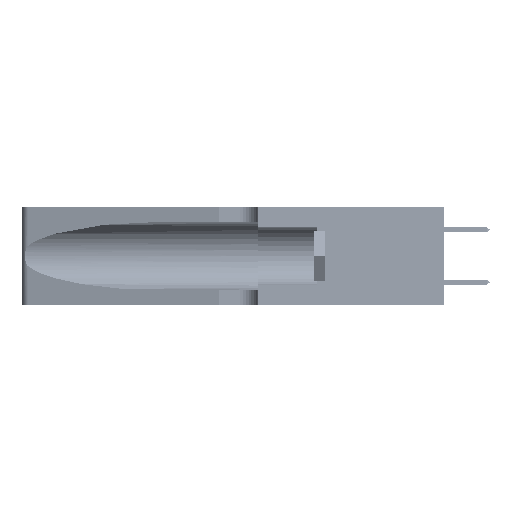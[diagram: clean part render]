
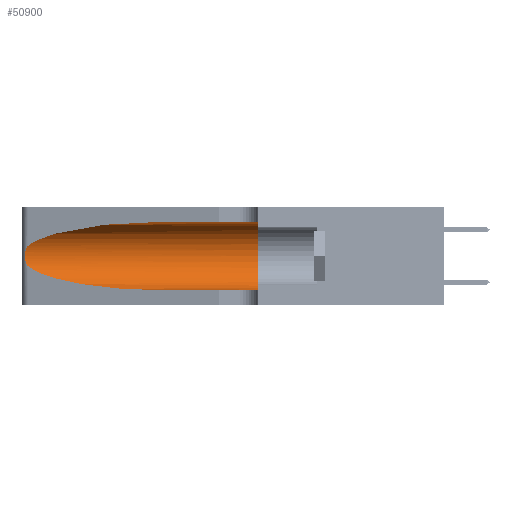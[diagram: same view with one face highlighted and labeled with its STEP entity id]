
A CAD part, left-side view. The second image highlights one B-rep face of the part: STEP entity #50900.
In plain terms, the highlighted cylindrical face has radius 3.308 mm (diameter 6.617 mm), a partial arc.
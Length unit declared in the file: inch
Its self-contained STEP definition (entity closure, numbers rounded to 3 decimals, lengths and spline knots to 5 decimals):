
#383 = CARTESIAN_POINT ( 'NONE',  ( 0.25487, 1.22718, 0.14631 ) ) ;
#480 = DIRECTION ( 'NONE',  ( 0., -1., 0. ) ) ;
#1795 = EDGE_CURVE ( 'NONE', #42013, #22346, #43611, .T. ) ;
#2925 = ORIENTED_EDGE ( 'NONE', *, *, #12198, .T. ) ;
#3217 = CARTESIAN_POINT ( 'NONE',  ( 0.25555, 1.22994, 0.2215 ) ) ;
#3364 = CARTESIAN_POINT ( 'NONE',  ( 0.25487, 1.22718, 0.22369 ) ) ;
#3569 = CARTESIAN_POINT ( 'NONE',  ( 0.25854, 1.2359, 0.20912 ) ) ;
#3576 = VERTEX_POINT ( 'NONE', #20899 ) ;
#4044 = CARTESIAN_POINT ( 'NONE',  ( 0.18966, 0.96281, 0.31525 ) ) ;
#4055 = LINE ( 'NONE', #19057, #10880 ) ;
#4656 = DIRECTION ( 'NONE',  ( 0., 0., -1. ) ) ;
#4986 =( BOUNDED_CURVE ( )  B_SPLINE_CURVE ( 3, ( #47479, #4044, #35626, #3364 ),
 .UNSPECIFIED., .F., .F. ) 
 B_SPLINE_CURVE_WITH_KNOTS ( ( 4, 4 ),
 ( 1.5708, 2.84003 ),
 .UNSPECIFIED. ) 
 CURVE ( )  GEOMETRIC_REPRESENTATION_ITEM ( )  RATIONAL_B_SPLINE_CURVE ( ( 1., 0.87, 0.87, 1. ) ) 
 REPRESENTATION_ITEM ( '' )  );
#7230 = CARTESIAN_POINT ( 'NONE',  ( 0.25487, 1.22718, 0.14631 ) ) ;
#7369 = CARTESIAN_POINT ( 'NONE',  ( 0.26075, 1.23896, 0.178 ) ) ;
#7662 = CYLINDRICAL_SURFACE ( 'NONE', #44489, 0.13025 ) ;
#8273 = CARTESIAN_POINT ( 'NONE',  ( 0.1305, 1.61858, 0.31525 ) ) ;
#9324 = EDGE_CURVE ( 'NONE', #22346, #3576, #16330, .T. ) ;
#10697 = CARTESIAN_POINT ( 'NONE',  ( 0.26017, 1.23833, 0.17102 ) ) ;
#10880 = VECTOR ( 'NONE', #31592, 39.37008 ) ;
#11208 = CARTESIAN_POINT ( 'NONE',  ( 0.25487, 1.22718, 0.14631 ) ) ;
#12198 = EDGE_CURVE ( 'NONE', #37770, #3576, #4055, .T. ) ;
#12504 = DIRECTION ( 'NONE',  ( 0., -1., 0. ) ) ;
#14277 =( BOUNDED_CURVE ( )  B_SPLINE_CURVE ( 3, ( #7230, #18972, #31347, #50701 ),
 .UNSPECIFIED., .F., .T. ) 
 B_SPLINE_CURVE_WITH_KNOTS ( ( 4, 4 ),
 ( 3.44316, 4.71239 ),
 .UNSPECIFIED. ) 
 CURVE ( )  GEOMETRIC_REPRESENTATION_ITEM ( )  RATIONAL_B_SPLINE_CURVE ( ( 1., 0.87, 0.87, 1. ) ) 
 REPRESENTATION_ITEM ( '' )  );
#15420 = CARTESIAN_POINT ( 'NONE',  ( 0.26075, 1.23896, 0.19203 ) ) ;
#16275 = ORIENTED_EDGE ( 'NONE', *, *, #34253, .T. ) ;
#16330 = CIRCLE ( 'NONE', #50431, 0.13025 ) ;
#18763 = CARTESIAN_POINT ( 'NONE',  ( 0.26018, 1.23835, 0.19895 ) ) ;
#18972 = CARTESIAN_POINT ( 'NONE',  ( 0.2373, 1.15595, 0.08982 ) ) ;
#19057 = CARTESIAN_POINT ( 'NONE',  ( 0.1305, 1.61858, 0.05475 ) ) ;
#20899 = CARTESIAN_POINT ( 'NONE',  ( 0.1305, 0.35, 0.05475 ) ) ;
#21268 = ORIENTED_EDGE ( 'NONE', *, *, #1795, .F. ) ;
#22346 = VERTEX_POINT ( 'NONE', #34883 ) ;
#22374 = ORIENTED_EDGE ( 'NONE', *, *, #42550, .T. ) ;
#26761 = CARTESIAN_POINT ( 'NONE',  ( 0.25639, 1.23186, 0.15144 ) ) ;
#27813 = CARTESIAN_POINT ( 'NONE',  ( 0.1305, 0.72297, 0.31525 ) ) ;
#27861 = CARTESIAN_POINT ( 'NONE',  ( 0.25487, 1.22718, 0.22369 ) ) ;
#29194 = VERTEX_POINT ( 'NONE', #383 ) ;
#30957 = CARTESIAN_POINT ( 'NONE',  ( 0.25787, 1.23484, 0.2124 ) ) ;
#31138 = CARTESIAN_POINT ( 'NONE',  ( 0.25789, 1.23486, 0.15765 ) ) ;
#31347 = CARTESIAN_POINT ( 'NONE',  ( 0.18966, 0.96281, 0.05475 ) ) ;
#31515 = EDGE_CURVE ( 'NONE', #29194, #37770, #14277, .T. ) ;
#31592 = DIRECTION ( 'NONE',  ( 0., -1., 0. ) ) ;
#33286 = FACE_OUTER_BOUND ( 'NONE', #48980, .T. ) ;
#33480 = B_SPLINE_CURVE_WITH_KNOTS ( 'NONE', 3,
 ( #43003, #3217, #42662, #30957, #3569, #18763, #15420, #7369, #10697, #38985, #31138, #26761, #35147, #11208 ),
 .UNSPECIFIED., .F., .F.,
 ( 4, 2, 2, 2, 2, 2, 4 ),
 ( 0., 0.00027, 0.00053, 0.00107, 0.0016, 0.00187, 0.00214 ),
 .UNSPECIFIED. ) ;
#33736 = DIRECTION ( 'NONE',  ( 0., 1., 0. ) ) ;
#34253 = EDGE_CURVE ( 'NONE', #50828, #29194, #33480, .T. ) ;
#34883 = CARTESIAN_POINT ( 'NONE',  ( 0.1305, 0.35, 0.31525 ) ) ;
#35147 = CARTESIAN_POINT ( 'NONE',  ( 0.25555, 1.22993, 0.14849 ) ) ;
#35626 = CARTESIAN_POINT ( 'NONE',  ( 0.2373, 1.15595, 0.28018 ) ) ;
#37377 = DIRECTION ( 'NONE',  ( 0., 0., 1. ) ) ;
#37770 = VERTEX_POINT ( 'NONE', #42036 ) ;
#38002 = ORIENTED_EDGE ( 'NONE', *, *, #9324, .F. ) ;
#38985 = CARTESIAN_POINT ( 'NONE',  ( 0.25856, 1.23593, 0.16098 ) ) ;
#41254 = CARTESIAN_POINT ( 'NONE',  ( 0.1305, 0.35, 0.185 ) ) ;
#41795 = VECTOR ( 'NONE', #480, 39.37008 ) ;
#42013 = VERTEX_POINT ( 'NONE', #27813 ) ;
#42036 = CARTESIAN_POINT ( 'NONE',  ( 0.1305, 0.72297, 0.05475 ) ) ;
#42550 = EDGE_CURVE ( 'NONE', #42013, #50828, #4986, .T. ) ;
#42662 = CARTESIAN_POINT ( 'NONE',  ( 0.25639, 1.23184, 0.21858 ) ) ;
#43003 = CARTESIAN_POINT ( 'NONE',  ( 0.25487, 1.22718, 0.22369 ) ) ;
#43611 = LINE ( 'NONE', #8273, #41795 ) ;
#44489 = AXIS2_PLACEMENT_3D ( 'NONE', #48267, #12504, #4656 ) ;
#47108 = ORIENTED_EDGE ( 'NONE', *, *, #31515, .T. ) ;
#47479 = CARTESIAN_POINT ( 'NONE',  ( 0.1305, 0.72297, 0.31525 ) ) ;
#48267 = CARTESIAN_POINT ( 'NONE',  ( 0.1305, 1.61858, 0.185 ) ) ;
#48980 = EDGE_LOOP ( 'NONE', ( #22374, #16275, #47108, #2925, #38002, #21268 ) ) ;
#50431 = AXIS2_PLACEMENT_3D ( 'NONE', #41254, #33736, #37377 ) ;
#50701 = CARTESIAN_POINT ( 'NONE',  ( 0.1305, 0.72297, 0.05475 ) ) ;
#50828 = VERTEX_POINT ( 'NONE', #27861 ) ;
#50900 = ADVANCED_FACE ( 'NONE', ( #33286 ), #7662, .F. ) ;
